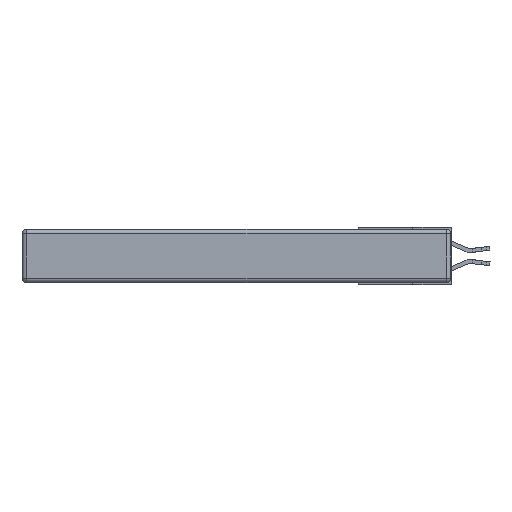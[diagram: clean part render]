
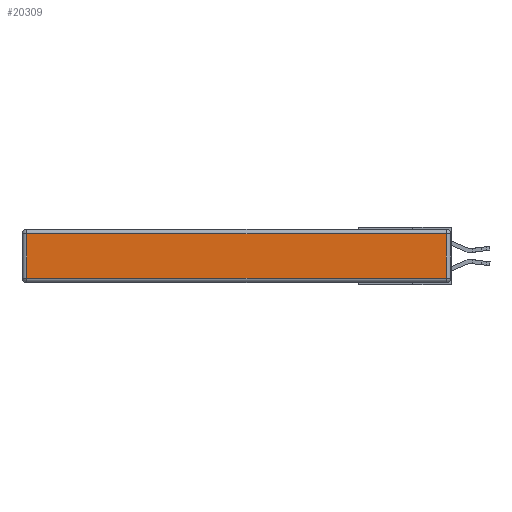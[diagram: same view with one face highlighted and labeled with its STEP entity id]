
A CAD part, left-side view. The second image highlights one B-rep face of the part: STEP entity #20309.
In plain terms, the highlighted planar face has unit normal (-1, 0, 0).
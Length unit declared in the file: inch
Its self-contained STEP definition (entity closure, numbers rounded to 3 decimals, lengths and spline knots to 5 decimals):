
#396 = CARTESIAN_POINT ( 'NONE',  ( 0., 2.72, -0.03 ) ) ;
#1617 = LINE ( 'NONE', #12677, #20927 ) ;
#4101 = FACE_OUTER_BOUND ( 'NONE', #23024, .T. ) ;
#4589 = ORIENTED_EDGE ( 'NONE', *, *, #7671, .T. ) ;
#5320 = DIRECTION ( 'NONE',  ( 0., 0., 1. ) ) ;
#6044 = DIRECTION ( 'NONE',  ( 0., 0., -1. ) ) ;
#7200 = VECTOR ( 'NONE', #5320, 39.37008 ) ;
#7671 = EDGE_CURVE ( 'NONE', #18183, #13467, #10847, .T. ) ;
#8040 = DIRECTION ( 'NONE',  ( -1., 0., 0. ) ) ;
#9013 = VECTOR ( 'NONE', #20493, 39.37008 ) ;
#9378 = CARTESIAN_POINT ( 'NONE',  ( 0., 2.72, -0.313 ) ) ;
#9925 = DIRECTION ( 'NONE',  ( 0., 0., 1. ) ) ;
#10443 = ORIENTED_EDGE ( 'NONE', *, *, #14487, .T. ) ;
#10847 = LINE ( 'NONE', #24262, #9013 ) ;
#11283 = CARTESIAN_POINT ( 'NONE',  ( 0., 0.03, -0.03 ) ) ;
#11800 = PLANE ( 'NONE',  #21849 ) ;
#12677 = CARTESIAN_POINT ( 'NONE',  ( 0., 0., -0.313 ) ) ;
#13169 = ORIENTED_EDGE ( 'NONE', *, *, #21988, .T. ) ;
#13467 = VERTEX_POINT ( 'NONE', #396 ) ;
#13661 = VERTEX_POINT ( 'NONE', #9378 ) ;
#14487 = EDGE_CURVE ( 'NONE', #18933, #18183, #22226, .T. ) ;
#14931 = CARTESIAN_POINT ( 'NONE',  ( 0., 0.03, -0.343 ) ) ;
#15815 = CARTESIAN_POINT ( 'NONE',  ( 0., 0., -0.343 ) ) ;
#15981 = EDGE_CURVE ( 'NONE', #13661, #18933, #1617, .T. ) ;
#17593 = ORIENTED_EDGE ( 'NONE', *, *, #15981, .T. ) ;
#18183 = VERTEX_POINT ( 'NONE', #11283 ) ;
#18933 = VERTEX_POINT ( 'NONE', #25071 ) ;
#19326 = DIRECTION ( 'NONE',  ( 0., -1., 0. ) ) ;
#19615 = VECTOR ( 'NONE', #6044, 39.37008 ) ;
#20309 = ADVANCED_FACE ( 'NONE', ( #4101 ), #11800, .T. ) ;
#20493 = DIRECTION ( 'NONE',  ( 0., 1., 0. ) ) ;
#20927 = VECTOR ( 'NONE', #19326, 39.37008 ) ;
#21803 = CARTESIAN_POINT ( 'NONE',  ( 0., 2.72, -0.343 ) ) ;
#21849 = AXIS2_PLACEMENT_3D ( 'NONE', #15815, #8040, #9925 ) ;
#21988 = EDGE_CURVE ( 'NONE', #13467, #13661, #24852, .T. ) ;
#22226 = LINE ( 'NONE', #14931, #7200 ) ;
#23024 = EDGE_LOOP ( 'NONE', ( #17593, #10443, #4589, #13169 ) ) ;
#24262 = CARTESIAN_POINT ( 'NONE',  ( 0., 2.75, -0.03 ) ) ;
#24852 = LINE ( 'NONE', #21803, #19615 ) ;
#25071 = CARTESIAN_POINT ( 'NONE',  ( 0., 0.03, -0.313 ) ) ;
